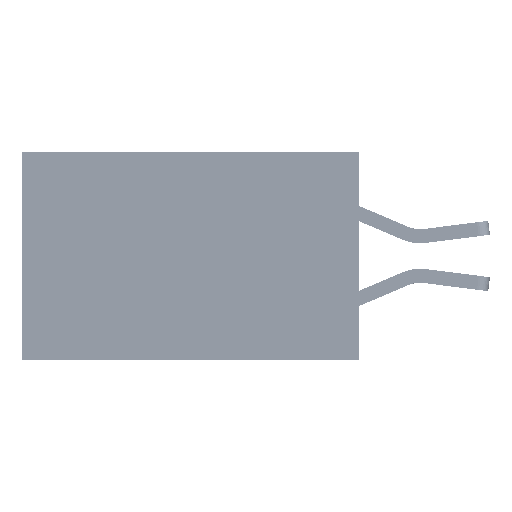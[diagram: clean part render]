
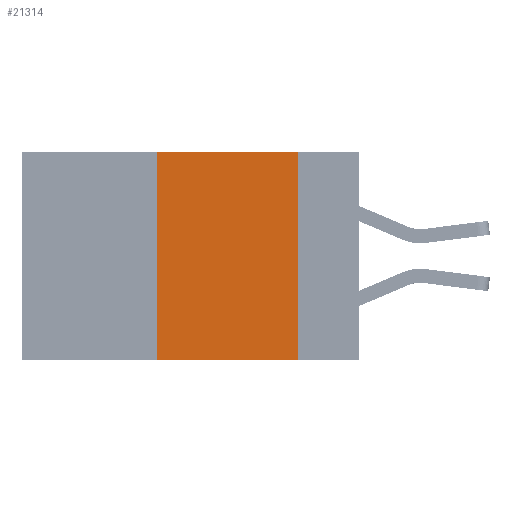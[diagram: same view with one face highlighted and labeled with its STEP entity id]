
A CAD part, left-side view. The second image highlights one B-rep face of the part: STEP entity #21314.
In plain terms, the highlighted planar face has unit normal (-1, 0, 0).
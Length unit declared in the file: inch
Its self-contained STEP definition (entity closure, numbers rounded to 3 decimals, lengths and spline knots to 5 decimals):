
#953 = CARTESIAN_POINT ( 'NONE',  ( 0., 0.6, 0. ) ) ;
#1130 = LINE ( 'NONE', #953, #35452 ) ;
#3869 = VERTEX_POINT ( 'NONE', #17475 ) ;
#4364 = CARTESIAN_POINT ( 'NONE',  ( 0., 0.36, 0. ) ) ;
#4427 = DIRECTION ( 'NONE',  ( 0., -1., 0. ) ) ;
#5982 = CARTESIAN_POINT ( 'NONE',  ( 0., 0.6, -0.37 ) ) ;
#7202 = EDGE_CURVE ( 'NONE', #28067, #3869, #1130, .T. ) ;
#7230 = VERTEX_POINT ( 'NONE', #24208 ) ;
#7986 = EDGE_CURVE ( 'NONE', #3869, #7230, #17109, .T. ) ;
#9983 = CARTESIAN_POINT ( 'NONE',  ( 0., 0.36, -0.37 ) ) ;
#10201 = ORIENTED_EDGE ( 'NONE', *, *, #32739, .F. ) ;
#14203 = VECTOR ( 'NONE', #27961, 39.37008 ) ;
#14772 = LINE ( 'NONE', #5982, #14203 ) ;
#16021 = FACE_OUTER_BOUND ( 'NONE', #39388, .T. ) ;
#17109 = LINE ( 'NONE', #30354, #30678 ) ;
#17475 = CARTESIAN_POINT ( 'NONE',  ( 0., 0.11, 0. ) ) ;
#18103 = CARTESIAN_POINT ( 'NONE',  ( 0., 0.6, 0. ) ) ;
#18321 = EDGE_CURVE ( 'NONE', #33119, #7230, #14772, .T. ) ;
#18542 = DIRECTION ( 'NONE',  ( 0., 0., -1. ) ) ;
#21314 = ADVANCED_FACE ( 'NONE', ( #16021 ), #31950, .F. ) ;
#24140 = DIRECTION ( 'NONE',  ( 0., 0., 1. ) ) ;
#24208 = CARTESIAN_POINT ( 'NONE',  ( 0., 0.11, -0.37 ) ) ;
#25282 = ORIENTED_EDGE ( 'NONE', *, *, #7986, .F. ) ;
#26633 = VECTOR ( 'NONE', #24140, 39.37008 ) ;
#27128 = LINE ( 'NONE', #4364, #26633 ) ;
#27860 = AXIS2_PLACEMENT_3D ( 'NONE', #18103, #41385, #18542 ) ;
#27961 = DIRECTION ( 'NONE',  ( 0., -1., 0. ) ) ;
#28067 = VERTEX_POINT ( 'NONE', #33251 ) ;
#30354 = CARTESIAN_POINT ( 'NONE',  ( 0., 0.11, 0. ) ) ;
#30678 = VECTOR ( 'NONE', #33671, 39.37008 ) ;
#31950 = PLANE ( 'NONE',  #27860 ) ;
#32739 = EDGE_CURVE ( 'NONE', #33119, #28067, #27128, .T. ) ;
#33119 = VERTEX_POINT ( 'NONE', #9983 ) ;
#33251 = CARTESIAN_POINT ( 'NONE',  ( 0., 0.36, 0. ) ) ;
#33671 = DIRECTION ( 'NONE',  ( 0., 0., -1. ) ) ;
#35452 = VECTOR ( 'NONE', #4427, 39.37008 ) ;
#36816 = ORIENTED_EDGE ( 'NONE', *, *, #7202, .F. ) ;
#39388 = EDGE_LOOP ( 'NONE', ( #25282, #36816, #10201, #42000 ) ) ;
#41385 = DIRECTION ( 'NONE',  ( 1., 0., 0. ) ) ;
#42000 = ORIENTED_EDGE ( 'NONE', *, *, #18321, .T. ) ;
